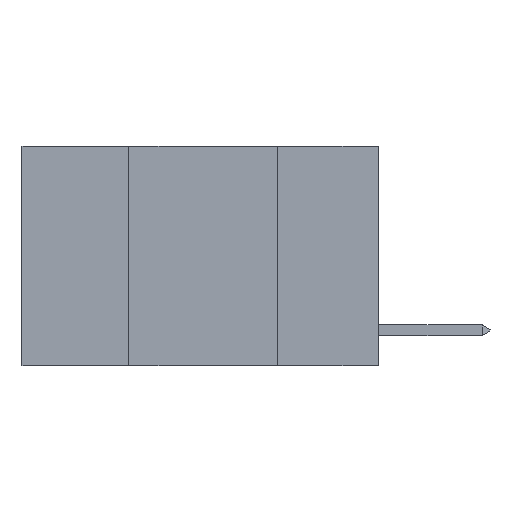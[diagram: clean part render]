
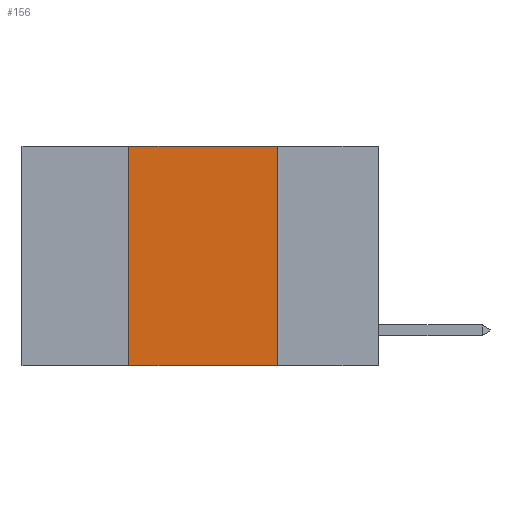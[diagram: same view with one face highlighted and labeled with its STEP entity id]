
A CAD part, left-side view. The second image highlights one B-rep face of the part: STEP entity #156.
In plain terms, the highlighted planar face has unit normal (-1, 0, 0).
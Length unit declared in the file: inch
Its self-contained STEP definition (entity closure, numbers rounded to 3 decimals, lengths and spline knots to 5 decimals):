
#93 = EDGE_CURVE ( 'NONE', #855, #2236, #10059, .T. ) ;
#113 = EDGE_CURVE ( 'NONE', #8724, #2265, #1015, .T. ) ;
#118 = EDGE_CURVE ( 'NONE', #8724, #2236, #3524, .T. ) ;
#156 = ADVANCED_FACE ( 'NONE', ( #5052 ), #6983, .F. ) ;
#263 = DIRECTION ( 'NONE',  ( 0., -1., 0. ) ) ;
#855 = VERTEX_POINT ( 'NONE', #8358 ) ;
#1015 = LINE ( 'NONE', #9898, #5765 ) ;
#1615 = VECTOR ( 'NONE', #4553, 39.37008 ) ;
#2236 = VERTEX_POINT ( 'NONE', #9021 ) ;
#2265 = VERTEX_POINT ( 'NONE', #3961 ) ;
#2540 = ORIENTED_EDGE ( 'NONE', *, *, #118, .T. ) ;
#2683 = CARTESIAN_POINT ( 'NONE',  ( 0., 0.6, 0. ) ) ;
#3164 = CARTESIAN_POINT ( 'NONE',  ( 0., 0.17, 0. ) ) ;
#3214 = VECTOR ( 'NONE', #263, 39.37008 ) ;
#3302 = DIRECTION ( 'NONE',  ( 0., 0., -1. ) ) ;
#3524 = LINE ( 'NONE', #6228, #3214 ) ;
#3575 = DIRECTION ( 'NONE',  ( 0., 0., -1. ) ) ;
#3961 = CARTESIAN_POINT ( 'NONE',  ( 0., 0.42, 0. ) ) ;
#4423 = CARTESIAN_POINT ( 'NONE',  ( 0., 0.6, 0. ) ) ;
#4553 = DIRECTION ( 'NONE',  ( 0., -1., 0. ) ) ;
#4709 = ORIENTED_EDGE ( 'NONE', *, *, #93, .F. ) ;
#4817 = EDGE_CURVE ( 'NONE', #2265, #855, #9854, .T. ) ;
#5052 = FACE_OUTER_BOUND ( 'NONE', #5679, .T. ) ;
#5481 = AXIS2_PLACEMENT_3D ( 'NONE', #4423, #8346, #3575 ) ;
#5679 = EDGE_LOOP ( 'NONE', ( #4709, #6707, #8554, #2540 ) ) ;
#5756 = CARTESIAN_POINT ( 'NONE',  ( 0., 0.42, -0.37 ) ) ;
#5765 = VECTOR ( 'NONE', #9682, 39.37008 ) ;
#6228 = CARTESIAN_POINT ( 'NONE',  ( 0., 0.6, -0.37 ) ) ;
#6438 = VECTOR ( 'NONE', #3302, 39.37008 ) ;
#6707 = ORIENTED_EDGE ( 'NONE', *, *, #4817, .F. ) ;
#6983 = PLANE ( 'NONE',  #5481 ) ;
#8346 = DIRECTION ( 'NONE',  ( 1., 0., 0. ) ) ;
#8358 = CARTESIAN_POINT ( 'NONE',  ( 0., 0.17, 0. ) ) ;
#8554 = ORIENTED_EDGE ( 'NONE', *, *, #113, .F. ) ;
#8724 = VERTEX_POINT ( 'NONE', #5756 ) ;
#9021 = CARTESIAN_POINT ( 'NONE',  ( 0., 0.17, -0.37 ) ) ;
#9682 = DIRECTION ( 'NONE',  ( 0., 0., 1. ) ) ;
#9854 = LINE ( 'NONE', #2683, #1615 ) ;
#9898 = CARTESIAN_POINT ( 'NONE',  ( 0., 0.42, 0. ) ) ;
#10059 = LINE ( 'NONE', #3164, #6438 ) ;
